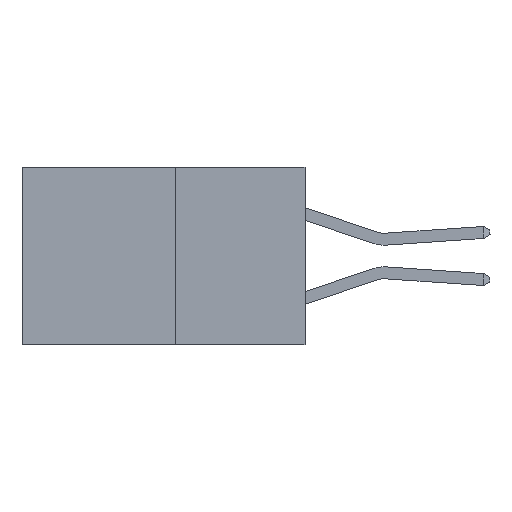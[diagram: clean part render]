
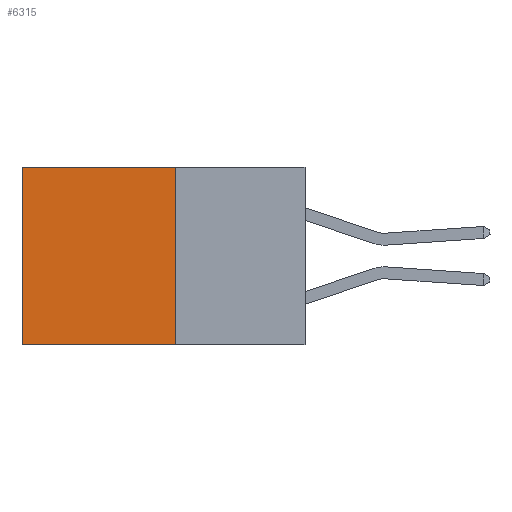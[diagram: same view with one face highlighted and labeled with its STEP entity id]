
A CAD part, left-side view. The second image highlights one B-rep face of the part: STEP entity #6315.
In plain terms, the highlighted planar face has unit normal (-1, 0, 0).
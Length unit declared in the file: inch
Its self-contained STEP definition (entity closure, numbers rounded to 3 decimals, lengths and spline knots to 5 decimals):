
#206 = EDGE_CURVE ( 'NONE', #1191, #8137, #11685, .T. ) ;
#1157 = CARTESIAN_POINT ( 'NONE',  ( 0.277, 0.27, -0.37 ) ) ;
#1191 = VERTEX_POINT ( 'NONE', #1157 ) ;
#1769 = VECTOR ( 'NONE', #5130, 39.37008 ) ;
#2777 = AXIS2_PLACEMENT_3D ( 'NONE', #12950, #14300, #14296 ) ;
#3196 = ORIENTED_EDGE ( 'NONE', *, *, #206, .F. ) ;
#3515 = DIRECTION ( 'NONE',  ( 0., 1., 0. ) ) ;
#4183 = VECTOR ( 'NONE', #3515, 39.37008 ) ;
#4241 = CARTESIAN_POINT ( 'NONE',  ( 0.277, 0.27, 0. ) ) ;
#4418 = ORIENTED_EDGE ( 'NONE', *, *, #16511, .T. ) ;
#4483 = ORIENTED_EDGE ( 'NONE', *, *, #17238, .T. ) ;
#4520 = DIRECTION ( 'NONE',  ( 0., 0., -1. ) ) ;
#5130 = DIRECTION ( 'NONE',  ( 0., 1., 0. ) ) ;
#6315 = ADVANCED_FACE ( 'NONE', ( #12652 ), #12975, .F. ) ;
#6712 = CARTESIAN_POINT ( 'NONE',  ( 0.277, 0.59, 0. ) ) ;
#6758 = LINE ( 'NONE', #17219, #18073 ) ;
#6813 = VECTOR ( 'NONE', #4520, 39.37008 ) ;
#7150 = CARTESIAN_POINT ( 'NONE',  ( 0.277, 0.27, -0.37 ) ) ;
#8137 = VERTEX_POINT ( 'NONE', #14202 ) ;
#8700 = DIRECTION ( 'NONE',  ( 0., 0., -1. ) ) ;
#10122 = LINE ( 'NONE', #12991, #6813 ) ;
#11417 = VERTEX_POINT ( 'NONE', #4241 ) ;
#11685 = LINE ( 'NONE', #7150, #4183 ) ;
#11958 = VERTEX_POINT ( 'NONE', #6712 ) ;
#12652 = FACE_OUTER_BOUND ( 'NONE', #12965, .T. ) ;
#12950 = CARTESIAN_POINT ( 'NONE',  ( 0.277, 0.27, -0.37 ) ) ;
#12965 = EDGE_LOOP ( 'NONE', ( #4418, #3196, #17738, #4483 ) ) ;
#12975 = PLANE ( 'NONE',  #2777 ) ;
#12991 = CARTESIAN_POINT ( 'NONE',  ( 0.277, 0.27, -0.37 ) ) ;
#13609 = CARTESIAN_POINT ( 'NONE',  ( 0.277, 0.27, 0. ) ) ;
#14202 = CARTESIAN_POINT ( 'NONE',  ( 0.277, 0.59, -0.37 ) ) ;
#14296 = DIRECTION ( 'NONE',  ( 0., 0., -1. ) ) ;
#14300 = DIRECTION ( 'NONE',  ( 1., 0., 0. ) ) ;
#15209 = EDGE_CURVE ( 'NONE', #11417, #1191, #10122, .T. ) ;
#16446 = LINE ( 'NONE', #13609, #1769 ) ;
#16511 = EDGE_CURVE ( 'NONE', #11958, #8137, #6758, .T. ) ;
#17219 = CARTESIAN_POINT ( 'NONE',  ( 0.277, 0.59, -0.37 ) ) ;
#17238 = EDGE_CURVE ( 'NONE', #11417, #11958, #16446, .T. ) ;
#17738 = ORIENTED_EDGE ( 'NONE', *, *, #15209, .F. ) ;
#18073 = VECTOR ( 'NONE', #8700, 39.37008 ) ;
